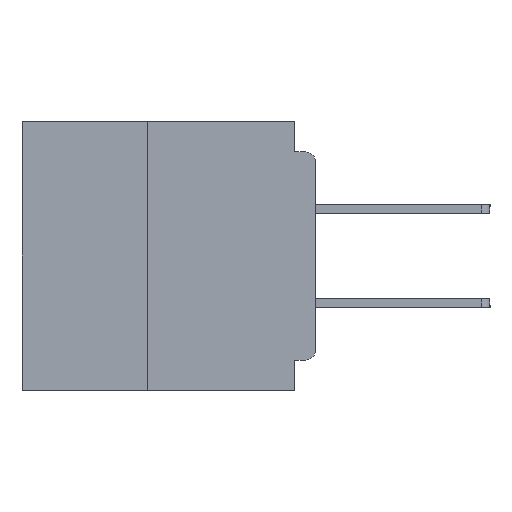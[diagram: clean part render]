
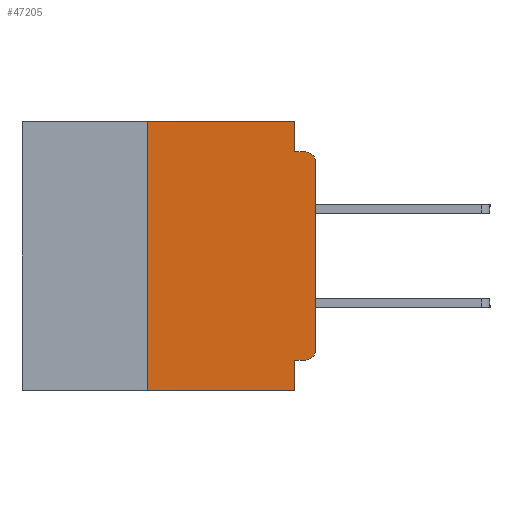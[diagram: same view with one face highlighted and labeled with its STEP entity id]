
A CAD part, left-side view. The second image highlights one B-rep face of the part: STEP entity #47205.
In plain terms, the highlighted planar face has unit normal (-1, 0, 0).
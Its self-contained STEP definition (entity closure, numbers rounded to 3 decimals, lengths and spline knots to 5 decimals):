
#365 = AXIS2_PLACEMENT_3D ( 'NONE', #56163, #27642, #60953 ) ;
#2149 = AXIS2_PLACEMENT_3D ( 'NONE', #23227, #42476, #13892 ) ;
#2591 = CARTESIAN_POINT ( 'NONE',  ( 0., 0., -0.045 ) ) ;
#3062 = EDGE_CURVE ( 'NONE', #15892, #59243, #20070, .T. ) ;
#3158 = LINE ( 'NONE', #10871, #39726 ) ;
#5458 = CARTESIAN_POINT ( 'NONE',  ( 0., 0.015, -0.355 ) ) ;
#6199 = EDGE_CURVE ( 'NONE', #10034, #15243, #11639, .T. ) ;
#8881 = LINE ( 'NONE', #41819, #20025 ) ;
#9259 = CARTESIAN_POINT ( 'NONE',  ( 0., 0.031, -0.045 ) ) ;
#9466 = ORIENTED_EDGE ( 'NONE', *, *, #12596, .T. ) ;
#10034 = VERTEX_POINT ( 'NONE', #5458 ) ;
#10269 = LINE ( 'NONE', #46130, #59414 ) ;
#10871 = CARTESIAN_POINT ( 'NONE',  ( 0., 0., 0. ) ) ;
#11639 = CIRCLE ( 'NONE', #365, 0.015 ) ;
#11969 = ORIENTED_EDGE ( 'NONE', *, *, #44217, .F. ) ;
#12596 = EDGE_CURVE ( 'NONE', #15243, #36970, #3158, .T. ) ;
#12757 = ORIENTED_EDGE ( 'NONE', *, *, #3062, .F. ) ;
#12971 = DIRECTION ( 'NONE',  ( 0., -1., 0. ) ) ;
#13892 = DIRECTION ( 'NONE',  ( 0., 0., -1. ) ) ;
#14594 = ORIENTED_EDGE ( 'NONE', *, *, #17886, .T. ) ;
#15243 = VERTEX_POINT ( 'NONE', #20551 ) ;
#15469 = CARTESIAN_POINT ( 'NONE',  ( 0., 0.015, -0.045 ) ) ;
#15892 = VERTEX_POINT ( 'NONE', #16273 ) ;
#16273 = CARTESIAN_POINT ( 'NONE',  ( 0., 0.031, 0. ) ) ;
#17886 = EDGE_CURVE ( 'NONE', #52882, #41539, #58456, .T. ) ;
#18087 = DIRECTION ( 'NONE',  ( -1., 0., 0. ) ) ;
#18535 = LINE ( 'NONE', #2591, #31262 ) ;
#19893 = CARTESIAN_POINT ( 'NONE',  ( 0., 0., -0.06 ) ) ;
#20025 = VECTOR ( 'NONE', #46615, 39.37008 ) ;
#20070 = LINE ( 'NONE', #29180, #32811 ) ;
#20551 = CARTESIAN_POINT ( 'NONE',  ( 0., 0., -0.34 ) ) ;
#22295 = CARTESIAN_POINT ( 'NONE',  ( 0., 0., -0.355 ) ) ;
#23209 = EDGE_CURVE ( 'NONE', #36970, #29778, #40320, .T. ) ;
#23227 = CARTESIAN_POINT ( 'NONE',  ( 0., 0.437, 0. ) ) ;
#23799 = EDGE_CURVE ( 'NONE', #59243, #29778, #18535, .T. ) ;
#24332 = CARTESIAN_POINT ( 'NONE',  ( 0., 0.031, -0.4 ) ) ;
#25682 = EDGE_CURVE ( 'NONE', #10034, #38163, #54209, .T. ) ;
#25785 = EDGE_LOOP ( 'NONE', ( #9466, #40334, #59792, #12757, #36142, #11969, #14594, #29234, #56312, #39844 ) ) ;
#27365 = VECTOR ( 'NONE', #41566, 39.37008 ) ;
#27642 = DIRECTION ( 'NONE',  ( -1., 0., 0. ) ) ;
#28440 = DIRECTION ( 'NONE',  ( 0., 0., 1. ) ) ;
#29180 = CARTESIAN_POINT ( 'NONE',  ( 0., 0.031, 0. ) ) ;
#29234 = ORIENTED_EDGE ( 'NONE', *, *, #31274, .F. ) ;
#29778 = VERTEX_POINT ( 'NONE', #15469 ) ;
#31262 = VECTOR ( 'NONE', #35943, 39.37008 ) ;
#31274 = EDGE_CURVE ( 'NONE', #38163, #41539, #8881, .T. ) ;
#31957 = FACE_OUTER_BOUND ( 'NONE', #25785, .T. ) ;
#32811 = VECTOR ( 'NONE', #52938, 39.37008 ) ;
#32926 = VECTOR ( 'NONE', #28440, 39.37008 ) ;
#34273 = VERTEX_POINT ( 'NONE', #59736 ) ;
#35943 = DIRECTION ( 'NONE',  ( 0., -1., 0. ) ) ;
#36142 = ORIENTED_EDGE ( 'NONE', *, *, #46336, .F. ) ;
#36970 = VERTEX_POINT ( 'NONE', #19893 ) ;
#38163 = VERTEX_POINT ( 'NONE', #56655 ) ;
#38171 = CARTESIAN_POINT ( 'NONE',  ( 0., 0.25, -0.4 ) ) ;
#39726 = VECTOR ( 'NONE', #53544, 39.37008 ) ;
#39844 = ORIENTED_EDGE ( 'NONE', *, *, #6199, .T. ) ;
#40320 = CIRCLE ( 'NONE', #58891, 0.015 ) ;
#40334 = ORIENTED_EDGE ( 'NONE', *, *, #23209, .T. ) ;
#41539 = VERTEX_POINT ( 'NONE', #24332 ) ;
#41566 = DIRECTION ( 'NONE',  ( 0., 1., 0. ) ) ;
#41819 = CARTESIAN_POINT ( 'NONE',  ( 0., 0.031, -0.4 ) ) ;
#42476 = DIRECTION ( 'NONE',  ( 1., 0., 0. ) ) ;
#44217 = EDGE_CURVE ( 'NONE', #52882, #34273, #45631, .T. ) ;
#45302 = DIRECTION ( 'NONE',  ( 0., -1., 0. ) ) ;
#45631 = LINE ( 'NONE', #57166, #32926 ) ;
#45861 = VECTOR ( 'NONE', #45302, 39.37008 ) ;
#46130 = CARTESIAN_POINT ( 'NONE',  ( 0., 0.437, 0. ) ) ;
#46336 = EDGE_CURVE ( 'NONE', #34273, #15892, #10269, .T. ) ;
#46615 = DIRECTION ( 'NONE',  ( 0., 0., -1. ) ) ;
#46727 = CARTESIAN_POINT ( 'NONE',  ( 0., 0.015, -0.06 ) ) ;
#47205 = ADVANCED_FACE ( 'NONE', ( #31957 ), #61374, .F. ) ;
#51441 = DIRECTION ( 'NONE',  ( 0., 0., -1. ) ) ;
#52882 = VERTEX_POINT ( 'NONE', #38171 ) ;
#52938 = DIRECTION ( 'NONE',  ( 0., 0., -1. ) ) ;
#53544 = DIRECTION ( 'NONE',  ( 0., 0., 1. ) ) ;
#54209 = LINE ( 'NONE', #22295, #27365 ) ;
#54603 = CARTESIAN_POINT ( 'NONE',  ( 0., 0.437, -0.4 ) ) ;
#56163 = CARTESIAN_POINT ( 'NONE',  ( 0., 0.015, -0.34 ) ) ;
#56312 = ORIENTED_EDGE ( 'NONE', *, *, #25682, .F. ) ;
#56655 = CARTESIAN_POINT ( 'NONE',  ( 0., 0.031, -0.355 ) ) ;
#57166 = CARTESIAN_POINT ( 'NONE',  ( 0., 0.25, -0.4 ) ) ;
#58456 = LINE ( 'NONE', #54603, #45861 ) ;
#58891 = AXIS2_PLACEMENT_3D ( 'NONE', #46727, #18087, #51441 ) ;
#59243 = VERTEX_POINT ( 'NONE', #9259 ) ;
#59414 = VECTOR ( 'NONE', #12971, 39.37008 ) ;
#59736 = CARTESIAN_POINT ( 'NONE',  ( 0., 0.25, 0. ) ) ;
#59792 = ORIENTED_EDGE ( 'NONE', *, *, #23799, .F. ) ;
#60953 = DIRECTION ( 'NONE',  ( 0., 0., -1. ) ) ;
#61374 = PLANE ( 'NONE',  #2149 ) ;
